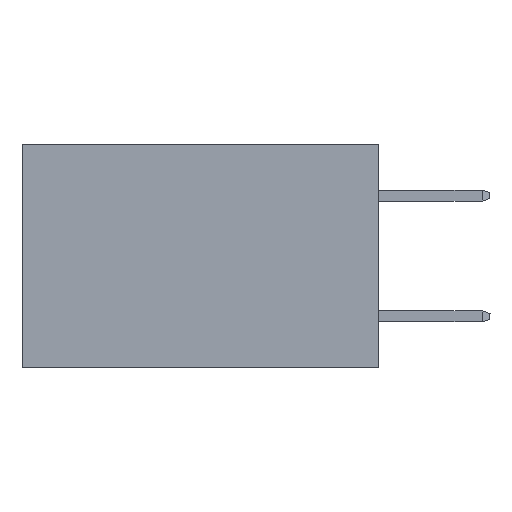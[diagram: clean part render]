
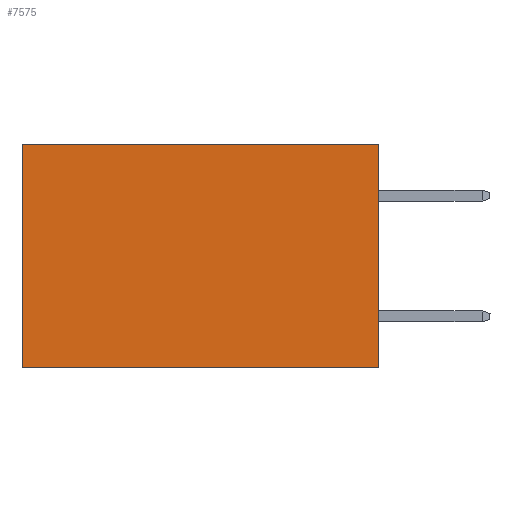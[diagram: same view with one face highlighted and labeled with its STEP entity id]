
A CAD part, left-side view. The second image highlights one B-rep face of the part: STEP entity #7575.
In plain terms, the highlighted planar face has unit normal (-1, 0, 0).
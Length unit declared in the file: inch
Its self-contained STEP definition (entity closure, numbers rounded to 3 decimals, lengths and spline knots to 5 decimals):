
#547 = LINE ( 'NONE', #27345, #7690 ) ;
#684 = FACE_OUTER_BOUND ( 'NONE', #6542, .T. ) ;
#1447 = CARTESIAN_POINT ( 'NONE',  ( 0.277, 0., 0. ) ) ;
#1507 = CARTESIAN_POINT ( 'NONE',  ( 0.277, 0., 0. ) ) ;
#3316 = VECTOR ( 'NONE', #4226, 39.37008 ) ;
#3477 = DIRECTION ( 'NONE',  ( 0., 0., -1. ) ) ;
#4226 = DIRECTION ( 'NONE',  ( 0., 1., 0. ) ) ;
#5374 = VERTEX_POINT ( 'NONE', #21989 ) ;
#5811 = EDGE_CURVE ( 'NONE', #28235, #5374, #6653, .T. ) ;
#6542 = EDGE_LOOP ( 'NONE', ( #10507, #24179, #10799, #9740 ) ) ;
#6653 = LINE ( 'NONE', #15796, #12931 ) ;
#6708 = VERTEX_POINT ( 'NONE', #1447 ) ;
#7575 = ADVANCED_FACE ( 'NONE', ( #684 ), #20321, .F. ) ;
#7690 = VECTOR ( 'NONE', #11467, 39.37008 ) ;
#7950 = VERTEX_POINT ( 'NONE', #13745 ) ;
#9369 = EDGE_CURVE ( 'NONE', #7950, #5374, #547, .T. ) ;
#9740 = ORIENTED_EDGE ( 'NONE', *, *, #16176, .T. ) ;
#9790 = DIRECTION ( 'NONE',  ( 0., 0., -1. ) ) ;
#10474 = LINE ( 'NONE', #1507, #3316 ) ;
#10507 = ORIENTED_EDGE ( 'NONE', *, *, #9369, .T. ) ;
#10799 = ORIENTED_EDGE ( 'NONE', *, *, #32386, .F. ) ;
#11467 = DIRECTION ( 'NONE',  ( 0., 0., -1. ) ) ;
#12931 = VECTOR ( 'NONE', #16118, 39.37008 ) ;
#13745 = CARTESIAN_POINT ( 'NONE',  ( 0.277, 0.59, 0. ) ) ;
#14137 = CARTESIAN_POINT ( 'NONE',  ( 0.277, 0., -0.37 ) ) ;
#15013 = CARTESIAN_POINT ( 'NONE',  ( 0.277, 0., -0.37 ) ) ;
#15796 = CARTESIAN_POINT ( 'NONE',  ( 0.277, 0., -0.37 ) ) ;
#16118 = DIRECTION ( 'NONE',  ( 0., 1., 0. ) ) ;
#16176 = EDGE_CURVE ( 'NONE', #6708, #7950, #10474, .T. ) ;
#18743 = CARTESIAN_POINT ( 'NONE',  ( 0.277, 0., -0.37 ) ) ;
#19911 = AXIS2_PLACEMENT_3D ( 'NONE', #15013, #25700, #9790 ) ;
#19997 = VECTOR ( 'NONE', #3477, 39.37008 ) ;
#20321 = PLANE ( 'NONE',  #19911 ) ;
#21989 = CARTESIAN_POINT ( 'NONE',  ( 0.277, 0.59, -0.37 ) ) ;
#24179 = ORIENTED_EDGE ( 'NONE', *, *, #5811, .F. ) ;
#25700 = DIRECTION ( 'NONE',  ( 1., 0., 0. ) ) ;
#27099 = LINE ( 'NONE', #14137, #19997 ) ;
#27345 = CARTESIAN_POINT ( 'NONE',  ( 0.277, 0.59, -0.37 ) ) ;
#28235 = VERTEX_POINT ( 'NONE', #18743 ) ;
#32386 = EDGE_CURVE ( 'NONE', #6708, #28235, #27099, .T. ) ;
